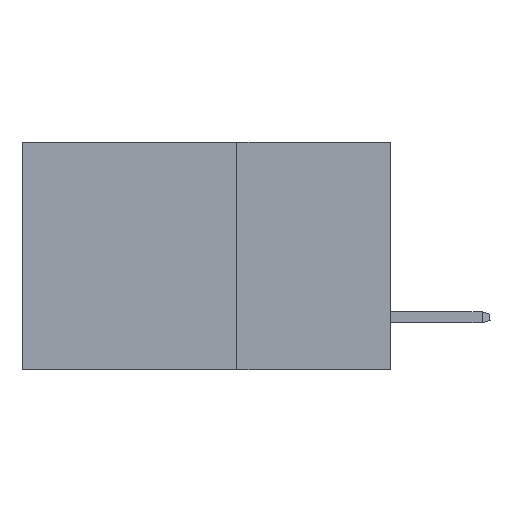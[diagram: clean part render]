
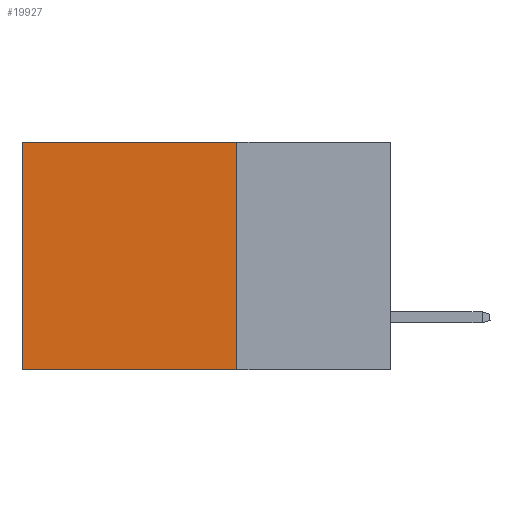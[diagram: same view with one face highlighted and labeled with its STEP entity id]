
A CAD part, left-side view. The second image highlights one B-rep face of the part: STEP entity #19927.
In plain terms, the highlighted planar face has unit normal (-1, 0, 0).
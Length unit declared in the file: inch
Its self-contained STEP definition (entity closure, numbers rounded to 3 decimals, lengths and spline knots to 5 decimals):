
#382 = CARTESIAN_POINT ( 'NONE',  ( 0.2875, 0.6, -0.37 ) ) ;
#936 = CARTESIAN_POINT ( 'NONE',  ( 0.2875, 0.25, 0. ) ) ;
#1511 = VECTOR ( 'NONE', #17727, 39.37008 ) ;
#1621 = PLANE ( 'NONE',  #19338 ) ;
#2519 = VERTEX_POINT ( 'NONE', #382 ) ;
#2542 = CARTESIAN_POINT ( 'NONE',  ( 0.2875, 0.25, -0.37 ) ) ;
#2808 = VERTEX_POINT ( 'NONE', #22194 ) ;
#3341 = ORIENTED_EDGE ( 'NONE', *, *, #7828, .F. ) ;
#3813 = LINE ( 'NONE', #22339, #16358 ) ;
#4806 = VECTOR ( 'NONE', #5245, 39.37008 ) ;
#5224 = EDGE_CURVE ( 'NONE', #26171, #2519, #24498, .T. ) ;
#5245 = DIRECTION ( 'NONE',  ( 0., 1., 0. ) ) ;
#5704 = CARTESIAN_POINT ( 'NONE',  ( 0.2875, 0.25, 0. ) ) ;
#5787 = EDGE_LOOP ( 'NONE', ( #27663, #27844, #3341, #8689 ) ) ;
#5973 = FACE_OUTER_BOUND ( 'NONE', #5787, .T. ) ;
#7828 = EDGE_CURVE ( 'NONE', #21820, #26171, #16288, .T. ) ;
#8689 = ORIENTED_EDGE ( 'NONE', *, *, #14575, .T. ) ;
#11621 = DIRECTION ( 'NONE',  ( 0., 0., -1. ) ) ;
#13814 = CARTESIAN_POINT ( 'NONE',  ( 0.2875, 0.25, 0. ) ) ;
#14561 = EDGE_CURVE ( 'NONE', #2808, #2519, #3813, .T. ) ;
#14575 = EDGE_CURVE ( 'NONE', #21820, #2808, #17702, .T. ) ;
#16288 = LINE ( 'NONE', #936, #25027 ) ;
#16358 = VECTOR ( 'NONE', #11621, 39.37008 ) ;
#16468 = CARTESIAN_POINT ( 'NONE',  ( 0.2875, 0.25, 0. ) ) ;
#17702 = LINE ( 'NONE', #13814, #4806 ) ;
#17727 = DIRECTION ( 'NONE',  ( 0., 1., 0. ) ) ;
#18572 = DIRECTION ( 'NONE',  ( 1., 0., 0. ) ) ;
#19338 = AXIS2_PLACEMENT_3D ( 'NONE', #5704, #18572, #22791 ) ;
#19927 = ADVANCED_FACE ( 'NONE', ( #5973 ), #1621, .F. ) ;
#21820 = VERTEX_POINT ( 'NONE', #16468 ) ;
#21865 = CARTESIAN_POINT ( 'NONE',  ( 0.2875, 0.25, -0.37 ) ) ;
#22194 = CARTESIAN_POINT ( 'NONE',  ( 0.2875, 0.6, 0. ) ) ;
#22339 = CARTESIAN_POINT ( 'NONE',  ( 0.2875, 0.6, 0. ) ) ;
#22791 = DIRECTION ( 'NONE',  ( 0., 0., -1. ) ) ;
#24498 = LINE ( 'NONE', #2542, #1511 ) ;
#25027 = VECTOR ( 'NONE', #26708, 39.37008 ) ;
#26171 = VERTEX_POINT ( 'NONE', #21865 ) ;
#26708 = DIRECTION ( 'NONE',  ( 0., 0., -1. ) ) ;
#27663 = ORIENTED_EDGE ( 'NONE', *, *, #14561, .T. ) ;
#27844 = ORIENTED_EDGE ( 'NONE', *, *, #5224, .F. ) ;
